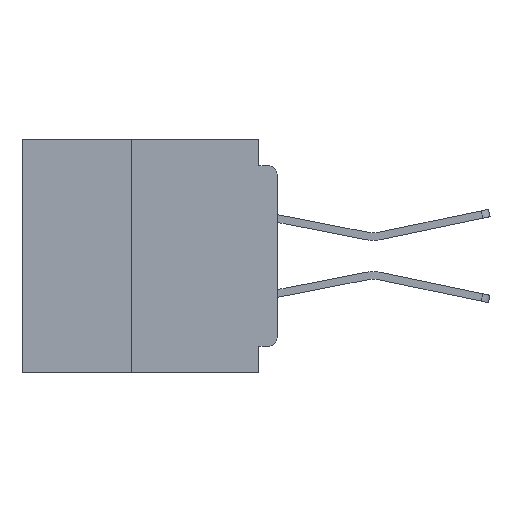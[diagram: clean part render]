
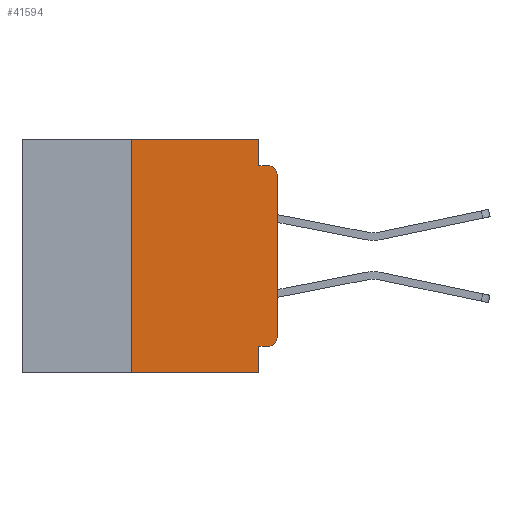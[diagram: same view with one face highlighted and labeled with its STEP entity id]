
A CAD part, left-side view. The second image highlights one B-rep face of the part: STEP entity #41594.
In plain terms, the highlighted planar face has unit normal (-1, 0, 0).
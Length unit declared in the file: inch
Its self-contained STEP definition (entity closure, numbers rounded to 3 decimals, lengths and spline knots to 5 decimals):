
#1644 = CARTESIAN_POINT ( 'NONE',  ( 0., 0.031, -0.355 ) ) ;
#2193 = LINE ( 'NONE', #18067, #36284 ) ;
#2921 = VERTEX_POINT ( 'NONE', #25927 ) ;
#3808 = CARTESIAN_POINT ( 'NONE',  ( 0., 0.015, -0.34 ) ) ;
#4388 = CARTESIAN_POINT ( 'NONE',  ( 0., 0., -0.045 ) ) ;
#4517 = AXIS2_PLACEMENT_3D ( 'NONE', #3808, #26957, #7125 ) ;
#5258 = FACE_OUTER_BOUND ( 'NONE', #37386, .T. ) ;
#5689 = EDGE_CURVE ( 'NONE', #31944, #14304, #14801, .T. ) ;
#6496 = PLANE ( 'NONE',  #29906 ) ;
#6993 = ORIENTED_EDGE ( 'NONE', *, *, #12249, .F. ) ;
#7125 = DIRECTION ( 'NONE',  ( 0., 0., -1. ) ) ;
#7633 = VECTOR ( 'NONE', #8612, 39.37008 ) ;
#8183 = CARTESIAN_POINT ( 'NONE',  ( 0., 0.015, -0.045 ) ) ;
#8612 = DIRECTION ( 'NONE',  ( 0., -1., 0. ) ) ;
#9698 = DIRECTION ( 'NONE',  ( 0., 0., -1. ) ) ;
#9803 = EDGE_CURVE ( 'NONE', #2921, #36733, #23434, .T. ) ;
#10209 = EDGE_CURVE ( 'NONE', #36733, #27734, #27541, .T. ) ;
#10301 = VECTOR ( 'NONE', #9698, 39.37008 ) ;
#10612 = VERTEX_POINT ( 'NONE', #1644 ) ;
#11292 = CARTESIAN_POINT ( 'NONE',  ( 0., 0., -0.355 ) ) ;
#11741 = EDGE_CURVE ( 'NONE', #18331, #10612, #35595, .T. ) ;
#12249 = EDGE_CURVE ( 'NONE', #10612, #42086, #32466, .T. ) ;
#12717 = VECTOR ( 'NONE', #33603, 39.37008 ) ;
#12863 = DIRECTION ( 'NONE',  ( -1., 0., 0. ) ) ;
#13200 = DIRECTION ( 'NONE',  ( 1., 0., 0. ) ) ;
#13919 = CARTESIAN_POINT ( 'NONE',  ( 0., 0., 0. ) ) ;
#14245 = VERTEX_POINT ( 'NONE', #20267 ) ;
#14304 = VERTEX_POINT ( 'NONE', #20557 ) ;
#14801 = LINE ( 'NONE', #33014, #12717 ) ;
#15061 = EDGE_CURVE ( 'NONE', #31276, #14245, #19382, .T. ) ;
#15845 = CARTESIAN_POINT ( 'NONE',  ( 0., 0., -0.06 ) ) ;
#16860 = CARTESIAN_POINT ( 'NONE',  ( 0., 0.031, 0. ) ) ;
#17110 = DIRECTION ( 'NONE',  ( 0., 0., 1. ) ) ;
#18067 = CARTESIAN_POINT ( 'NONE',  ( 0., 0.437, 0. ) ) ;
#18331 = VERTEX_POINT ( 'NONE', #26528 ) ;
#18909 = CIRCLE ( 'NONE', #4517, 0.015 ) ;
#19382 = LINE ( 'NONE', #34437, #35844 ) ;
#20083 = ORIENTED_EDGE ( 'NONE', *, *, #32321, .T. ) ;
#20267 = CARTESIAN_POINT ( 'NONE',  ( 0., 0.031, -0.045 ) ) ;
#20557 = CARTESIAN_POINT ( 'NONE',  ( 0., 0.25, 0. ) ) ;
#21359 = DIRECTION ( 'NONE',  ( 0., -1., 0. ) ) ;
#21549 = ORIENTED_EDGE ( 'NONE', *, *, #10209, .T. ) ;
#22083 = CARTESIAN_POINT ( 'NONE',  ( 0., 0.031, -0.4 ) ) ;
#23006 = CARTESIAN_POINT ( 'NONE',  ( 0., 0.437, 0. ) ) ;
#23161 = ORIENTED_EDGE ( 'NONE', *, *, #25890, .F. ) ;
#23367 = VECTOR ( 'NONE', #24210, 39.37008 ) ;
#23434 = LINE ( 'NONE', #13919, #39890 ) ;
#24174 = ORIENTED_EDGE ( 'NONE', *, *, #25318, .F. ) ;
#24210 = DIRECTION ( 'NONE',  ( 0., -1., 0. ) ) ;
#24423 = LINE ( 'NONE', #4388, #23367 ) ;
#25318 = EDGE_CURVE ( 'NONE', #14304, #31276, #2193, .T. ) ;
#25786 = AXIS2_PLACEMENT_3D ( 'NONE', #32584, #12863, #35893 ) ;
#25890 = EDGE_CURVE ( 'NONE', #14245, #27734, #24423, .T. ) ;
#25927 = CARTESIAN_POINT ( 'NONE',  ( 0., 0., -0.34 ) ) ;
#26304 = LINE ( 'NONE', #31724, #7633 ) ;
#26528 = CARTESIAN_POINT ( 'NONE',  ( 0., 0.015, -0.355 ) ) ;
#26957 = DIRECTION ( 'NONE',  ( -1., 0., 0. ) ) ;
#27541 = CIRCLE ( 'NONE', #25786, 0.015 ) ;
#27734 = VERTEX_POINT ( 'NONE', #8183 ) ;
#28484 = ORIENTED_EDGE ( 'NONE', *, *, #9803, .T. ) ;
#29237 = ORIENTED_EDGE ( 'NONE', *, *, #11741, .F. ) ;
#29500 = CARTESIAN_POINT ( 'NONE',  ( 0., 0.031, -0.4 ) ) ;
#29906 = AXIS2_PLACEMENT_3D ( 'NONE', #23006, #13200, #36236 ) ;
#30652 = ORIENTED_EDGE ( 'NONE', *, *, #15061, .F. ) ;
#31276 = VERTEX_POINT ( 'NONE', #16860 ) ;
#31724 = CARTESIAN_POINT ( 'NONE',  ( 0., 0.437, -0.4 ) ) ;
#31944 = VERTEX_POINT ( 'NONE', #39796 ) ;
#32321 = EDGE_CURVE ( 'NONE', #31944, #42086, #26304, .T. ) ;
#32466 = LINE ( 'NONE', #29500, #10301 ) ;
#32584 = CARTESIAN_POINT ( 'NONE',  ( 0., 0.015, -0.06 ) ) ;
#33014 = CARTESIAN_POINT ( 'NONE',  ( 0., 0.25, -0.4 ) ) ;
#33603 = DIRECTION ( 'NONE',  ( 0., 0., 1. ) ) ;
#34437 = CARTESIAN_POINT ( 'NONE',  ( 0., 0.031, 0. ) ) ;
#34572 = VECTOR ( 'NONE', #37675, 39.37008 ) ;
#34715 = EDGE_CURVE ( 'NONE', #18331, #2921, #18909, .T. ) ;
#35330 = ORIENTED_EDGE ( 'NONE', *, *, #34715, .T. ) ;
#35595 = LINE ( 'NONE', #11292, #34572 ) ;
#35844 = VECTOR ( 'NONE', #37758, 39.37008 ) ;
#35893 = DIRECTION ( 'NONE',  ( 0., 0., -1. ) ) ;
#36236 = DIRECTION ( 'NONE',  ( 0., 0., -1. ) ) ;
#36284 = VECTOR ( 'NONE', #21359, 39.37008 ) ;
#36733 = VERTEX_POINT ( 'NONE', #15845 ) ;
#36933 = ORIENTED_EDGE ( 'NONE', *, *, #5689, .F. ) ;
#37386 = EDGE_LOOP ( 'NONE', ( #28484, #21549, #23161, #30652, #24174, #36933, #20083, #6993, #29237, #35330 ) ) ;
#37675 = DIRECTION ( 'NONE',  ( 0., 1., 0. ) ) ;
#37758 = DIRECTION ( 'NONE',  ( 0., 0., -1. ) ) ;
#39796 = CARTESIAN_POINT ( 'NONE',  ( 0., 0.25, -0.4 ) ) ;
#39890 = VECTOR ( 'NONE', #17110, 39.37008 ) ;
#41594 = ADVANCED_FACE ( 'NONE', ( #5258 ), #6496, .F. ) ;
#42086 = VERTEX_POINT ( 'NONE', #22083 ) ;
